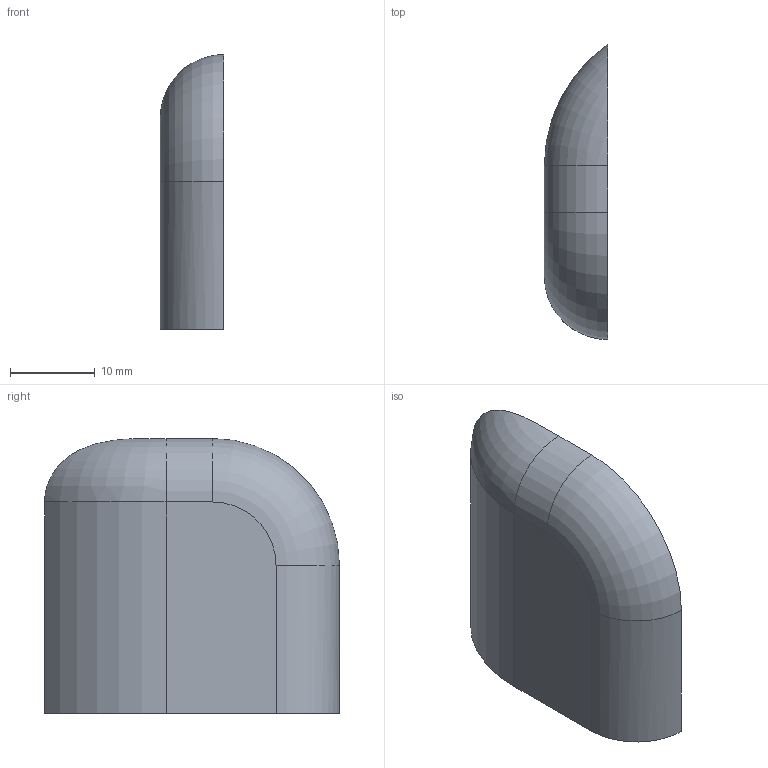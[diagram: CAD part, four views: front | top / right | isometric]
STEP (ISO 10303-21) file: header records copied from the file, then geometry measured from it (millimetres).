
FILE_DESCRIPTION (( 'STEP AP214' ), '1' );
FILE_NAME ('Side_Extension_Left.STEP', '2014-02-20T01:34:59', ( '' ), ( '' ), 'SwSTEP 2.0', 'SolidWorks 2013', '' );
FILE_SCHEMA (( 'AUTOMOTIVE_DESIGN' ));
Length unit declared in the file: millimetre
Products named in the file (1): Side_Extension_Left
Bounding box: 7.5 x 34.86 x 32.5 mm (x, y, z)
Volume: 6195.7 mm3; surface area: 2816.2 mm2
Topology: 1 solids, 1 shells, 20 faces, 41 edges, 27 vertices
Faces by surface type: cylinder 10, plane 7, torus 2, bspline 1
Entity records: 615 total; most frequent: CARTESIAN_POINT 141, DIRECTION 101, ORIENTED_EDGE 82, AXIS2_PLACEMENT_3D 43, EDGE_CURVE 41, VERTEX_POINT 27, EDGE_LOOP 24, CIRCLE 23
